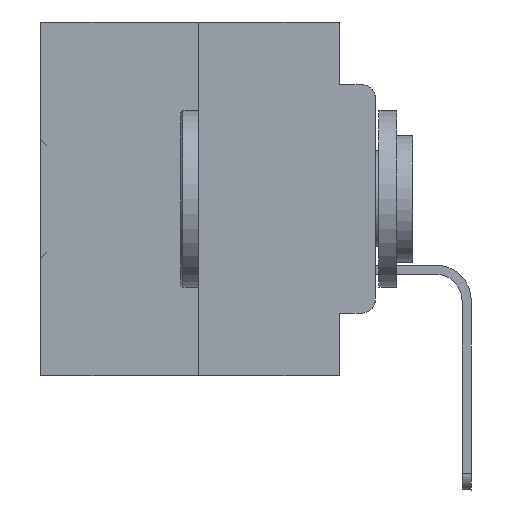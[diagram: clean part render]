
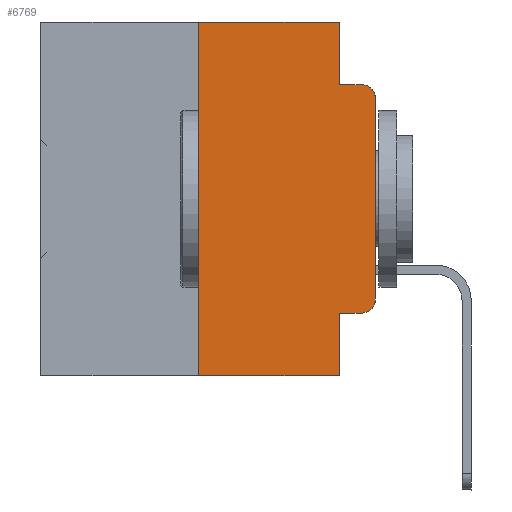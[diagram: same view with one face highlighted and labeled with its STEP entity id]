
A CAD part, left-side view. The second image highlights one B-rep face of the part: STEP entity #6769.
In plain terms, the highlighted planar face has unit normal (-1, 0, 0).
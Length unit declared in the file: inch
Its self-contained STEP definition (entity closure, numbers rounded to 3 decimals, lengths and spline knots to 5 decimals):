
#269 = CARTESIAN_POINT ( 'NONE',  ( 0., 0.02, -0.3915 ) ) ;
#874 = DIRECTION ( 'NONE',  ( 0., 0., -1. ) ) ;
#1240 = LINE ( 'NONE', #26262, #8410 ) ;
#1899 = EDGE_CURVE ( 'NONE', #17800, #10660, #16695, .T. ) ;
#1943 = ORIENTED_EDGE ( 'NONE', *, *, #35707, .T. ) ;
#1978 = LINE ( 'NONE', #17033, #3758 ) ;
#2629 = VECTOR ( 'NONE', #3156, 39.37008 ) ;
#3156 = DIRECTION ( 'NONE',  ( 0., 0., 1. ) ) ;
#3524 = CARTESIAN_POINT ( 'NONE',  ( 0., 0.25, 0. ) ) ;
#3758 = VECTOR ( 'NONE', #23019, 39.37008 ) ;
#4250 = DIRECTION ( 'NONE',  ( 0., 0., 1. ) ) ;
#4323 = CARTESIAN_POINT ( 'NONE',  ( 0., 0.051, -0.5 ) ) ;
#4513 = ORIENTED_EDGE ( 'NONE', *, *, #8773, .F. ) ;
#4567 = CARTESIAN_POINT ( 'NONE',  ( 0., 0.473, 0. ) ) ;
#4808 = VECTOR ( 'NONE', #874, 39.37008 ) ;
#4843 = VECTOR ( 'NONE', #6935, 39.37008 ) ;
#5376 = VERTEX_POINT ( 'NONE', #29898 ) ;
#5889 = AXIS2_PLACEMENT_3D ( 'NONE', #26160, #26674, #11880 ) ;
#6257 = ORIENTED_EDGE ( 'NONE', *, *, #16845, .F. ) ;
#6769 = ADVANCED_FACE ( 'NONE', ( #27087 ), #20847, .F. ) ;
#6835 = VERTEX_POINT ( 'NONE', #4323 ) ;
#6846 = VERTEX_POINT ( 'NONE', #7220 ) ;
#6935 = DIRECTION ( 'NONE',  ( 0., 0., -1. ) ) ;
#7220 = CARTESIAN_POINT ( 'NONE',  ( 0., 0.051, -0.0885 ) ) ;
#7338 = CARTESIAN_POINT ( 'NONE',  ( 0., 0.02, -0.4115 ) ) ;
#8410 = VECTOR ( 'NONE', #17731, 39.37008 ) ;
#8691 = ORIENTED_EDGE ( 'NONE', *, *, #10794, .F. ) ;
#8773 = EDGE_CURVE ( 'NONE', #15758, #37034, #15206, .T. ) ;
#8846 = DIRECTION ( 'NONE',  ( 0., -1., 0. ) ) ;
#9282 = EDGE_CURVE ( 'NONE', #37034, #6846, #18762, .T. ) ;
#9898 = DIRECTION ( 'NONE',  ( -1., 0., 0. ) ) ;
#10027 = DIRECTION ( 'NONE',  ( 0., 0., -1. ) ) ;
#10605 = LINE ( 'NONE', #24460, #30771 ) ;
#10660 = VERTEX_POINT ( 'NONE', #28739 ) ;
#10794 = EDGE_CURVE ( 'NONE', #27126, #15758, #28231, .T. ) ;
#10935 = ORIENTED_EDGE ( 'NONE', *, *, #24567, .T. ) ;
#11023 = ORIENTED_EDGE ( 'NONE', *, *, #21437, .F. ) ;
#11880 = DIRECTION ( 'NONE',  ( 0., 0., -1. ) ) ;
#12096 = ORIENTED_EDGE ( 'NONE', *, *, #21039, .T. ) ;
#12370 = VECTOR ( 'NONE', #8846, 39.37008 ) ;
#12829 = CARTESIAN_POINT ( 'NONE',  ( 0., 0.051, 0. ) ) ;
#12912 = CARTESIAN_POINT ( 'NONE',  ( 0., 0.02, -0.1085 ) ) ;
#13531 = CARTESIAN_POINT ( 'NONE',  ( 0., 0., -0.1085 ) ) ;
#14342 = ORIENTED_EDGE ( 'NONE', *, *, #9282, .F. ) ;
#15206 = LINE ( 'NONE', #4567, #28681 ) ;
#15604 = AXIS2_PLACEMENT_3D ( 'NONE', #269, #28614, #17329 ) ;
#15758 = VERTEX_POINT ( 'NONE', #35169 ) ;
#16695 = CIRCLE ( 'NONE', #15604, 0.02 ) ;
#16700 = VERTEX_POINT ( 'NONE', #13531 ) ;
#16845 = EDGE_CURVE ( 'NONE', #6846, #22201, #1978, .T. ) ;
#17033 = CARTESIAN_POINT ( 'NONE',  ( 0., 0.051, -0.0885 ) ) ;
#17243 = CIRCLE ( 'NONE', #22748, 0.02 ) ;
#17329 = DIRECTION ( 'NONE',  ( 0., 0., -1. ) ) ;
#17731 = DIRECTION ( 'NONE',  ( 0., -1., 0. ) ) ;
#17800 = VERTEX_POINT ( 'NONE', #7338 ) ;
#18762 = LINE ( 'NONE', #35652, #4843 ) ;
#20847 = PLANE ( 'NONE',  #5889 ) ;
#21039 = EDGE_CURVE ( 'NONE', #5376, #17800, #1240, .T. ) ;
#21437 = EDGE_CURVE ( 'NONE', #5376, #6835, #36638, .T. ) ;
#22121 = ORIENTED_EDGE ( 'NONE', *, *, #23819, .T. ) ;
#22201 = VERTEX_POINT ( 'NONE', #36064 ) ;
#22748 = AXIS2_PLACEMENT_3D ( 'NONE', #12912, #9898, #10027 ) ;
#23019 = DIRECTION ( 'NONE',  ( 0., -1., 0. ) ) ;
#23819 = EDGE_CURVE ( 'NONE', #27126, #6835, #31194, .T. ) ;
#24460 = CARTESIAN_POINT ( 'NONE',  ( 0., 0., 0. ) ) ;
#24567 = EDGE_CURVE ( 'NONE', #16700, #22201, #17243, .T. ) ;
#26160 = CARTESIAN_POINT ( 'NONE',  ( 0., 0.473, 0. ) ) ;
#26262 = CARTESIAN_POINT ( 'NONE',  ( 0., 0.051, -0.4115 ) ) ;
#26674 = DIRECTION ( 'NONE',  ( 1., 0., 0. ) ) ;
#26966 = ORIENTED_EDGE ( 'NONE', *, *, #1899, .T. ) ;
#27087 = FACE_OUTER_BOUND ( 'NONE', #32465, .T. ) ;
#27126 = VERTEX_POINT ( 'NONE', #33623 ) ;
#28231 = LINE ( 'NONE', #3524, #2629 ) ;
#28614 = DIRECTION ( 'NONE',  ( -1., 0., 0. ) ) ;
#28681 = VECTOR ( 'NONE', #33373, 39.37008 ) ;
#28739 = CARTESIAN_POINT ( 'NONE',  ( 0., 0., -0.3915 ) ) ;
#29840 = CARTESIAN_POINT ( 'NONE',  ( 0., 0.051, 0. ) ) ;
#29898 = CARTESIAN_POINT ( 'NONE',  ( 0., 0.051, -0.4115 ) ) ;
#30771 = VECTOR ( 'NONE', #4250, 39.37008 ) ;
#31194 = LINE ( 'NONE', #32145, #12370 ) ;
#32145 = CARTESIAN_POINT ( 'NONE',  ( 0., 0.473, -0.5 ) ) ;
#32465 = EDGE_LOOP ( 'NONE', ( #1943, #10935, #6257, #14342, #4513, #8691, #22121, #11023, #12096, #26966 ) ) ;
#33373 = DIRECTION ( 'NONE',  ( 0., -1., 0. ) ) ;
#33623 = CARTESIAN_POINT ( 'NONE',  ( 0., 0.25, -0.5 ) ) ;
#35169 = CARTESIAN_POINT ( 'NONE',  ( 0., 0.25, 0. ) ) ;
#35652 = CARTESIAN_POINT ( 'NONE',  ( 0., 0.051, 0. ) ) ;
#35707 = EDGE_CURVE ( 'NONE', #10660, #16700, #10605, .T. ) ;
#36064 = CARTESIAN_POINT ( 'NONE',  ( 0., 0.02, -0.0885 ) ) ;
#36638 = LINE ( 'NONE', #29840, #4808 ) ;
#37034 = VERTEX_POINT ( 'NONE', #12829 ) ;
